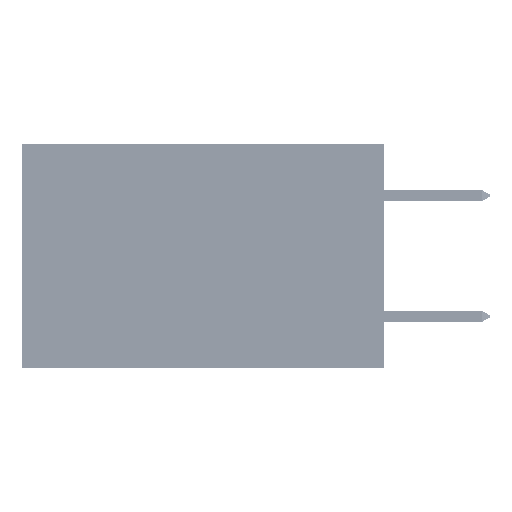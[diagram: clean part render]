
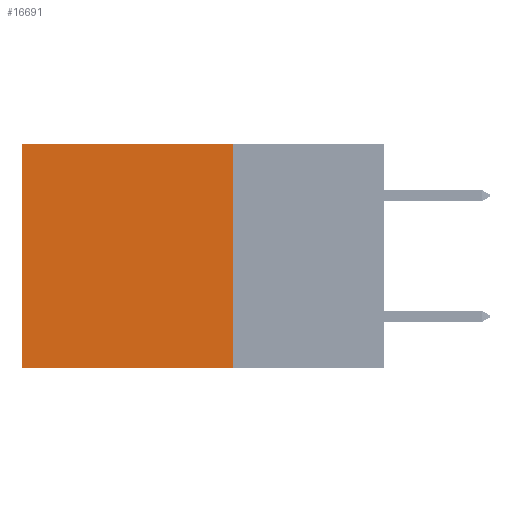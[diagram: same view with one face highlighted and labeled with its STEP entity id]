
A CAD part, left-side view. The second image highlights one B-rep face of the part: STEP entity #16691.
In plain terms, the highlighted planar face has unit normal (-1, 0, 0).
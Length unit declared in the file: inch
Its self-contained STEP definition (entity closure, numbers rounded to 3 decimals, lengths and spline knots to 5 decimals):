
#78 = AXIS2_PLACEMENT_3D ( 'NONE', #23435, #6527, #24195 ) ;
#445 = CARTESIAN_POINT ( 'NONE',  ( 0.2875, 0.25, 0. ) ) ;
#767 = CARTESIAN_POINT ( 'NONE',  ( 0.2875, 0.6, 0. ) ) ;
#1014 = LINE ( 'NONE', #4599, #7202 ) ;
#2412 = VERTEX_POINT ( 'NONE', #12726 ) ;
#4107 = CARTESIAN_POINT ( 'NONE',  ( 0.2875, 0.25, -0.37 ) ) ;
#4599 = CARTESIAN_POINT ( 'NONE',  ( 0.2875, 0.25, 0. ) ) ;
#6527 = DIRECTION ( 'NONE',  ( 1., 0., 0. ) ) ;
#7202 = VECTOR ( 'NONE', #7899, 39.37008 ) ;
#7899 = DIRECTION ( 'NONE',  ( 0., 1., 0. ) ) ;
#8145 = DIRECTION ( 'NONE',  ( 0., 1., 0. ) ) ;
#10493 = EDGE_CURVE ( 'NONE', #32682, #23405, #43668, .T. ) ;
#12195 = EDGE_CURVE ( 'NONE', #2412, #32682, #46380, .T. ) ;
#12483 = DIRECTION ( 'NONE',  ( 0., 0., -1. ) ) ;
#12726 = CARTESIAN_POINT ( 'NONE',  ( 0.2875, 0.25, 0. ) ) ;
#14384 = EDGE_CURVE ( 'NONE', #2412, #43605, #1014, .T. ) ;
#15389 = ORIENTED_EDGE ( 'NONE', *, *, #14384, .T. ) ;
#16691 = ADVANCED_FACE ( 'NONE', ( #23680 ), #38782, .F. ) ;
#19256 = VECTOR ( 'NONE', #8145, 39.37008 ) ;
#19413 = EDGE_CURVE ( 'NONE', #43605, #23405, #35487, .T. ) ;
#19549 = DIRECTION ( 'NONE',  ( 0., 0., -1. ) ) ;
#23181 = ORIENTED_EDGE ( 'NONE', *, *, #12195, .F. ) ;
#23293 = CARTESIAN_POINT ( 'NONE',  ( 0.2875, 0.6, 0. ) ) ;
#23405 = VERTEX_POINT ( 'NONE', #43387 ) ;
#23435 = CARTESIAN_POINT ( 'NONE',  ( 0.2875, 0.25, 0. ) ) ;
#23680 = FACE_OUTER_BOUND ( 'NONE', #37955, .T. ) ;
#24195 = DIRECTION ( 'NONE',  ( 0., 0., -1. ) ) ;
#24753 = ORIENTED_EDGE ( 'NONE', *, *, #19413, .T. ) ;
#30033 = VECTOR ( 'NONE', #19549, 39.37008 ) ;
#32682 = VERTEX_POINT ( 'NONE', #4107 ) ;
#33538 = VECTOR ( 'NONE', #12483, 39.37008 ) ;
#35487 = LINE ( 'NONE', #767, #33538 ) ;
#37955 = EDGE_LOOP ( 'NONE', ( #24753, #42233, #23181, #15389 ) ) ;
#38782 = PLANE ( 'NONE',  #78 ) ;
#39803 = CARTESIAN_POINT ( 'NONE',  ( 0.2875, 0.25, -0.37 ) ) ;
#42233 = ORIENTED_EDGE ( 'NONE', *, *, #10493, .F. ) ;
#43387 = CARTESIAN_POINT ( 'NONE',  ( 0.2875, 0.6, -0.37 ) ) ;
#43605 = VERTEX_POINT ( 'NONE', #23293 ) ;
#43668 = LINE ( 'NONE', #39803, #19256 ) ;
#46380 = LINE ( 'NONE', #445, #30033 ) ;
